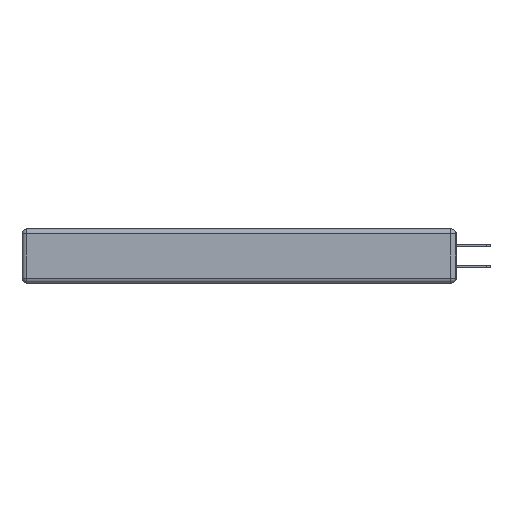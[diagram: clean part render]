
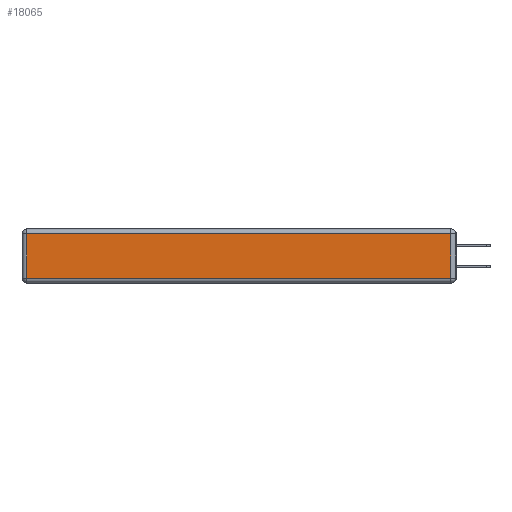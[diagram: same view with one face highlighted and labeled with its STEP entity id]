
A CAD part, left-side view. The second image highlights one B-rep face of the part: STEP entity #18065.
In plain terms, the highlighted planar face has unit normal (-1, 0, 0).
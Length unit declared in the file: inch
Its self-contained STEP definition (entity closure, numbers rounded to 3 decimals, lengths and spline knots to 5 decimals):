
#1673 = EDGE_LOOP ( 'NONE', ( #3307, #16689, #12419, #11632 ) ) ;
#2070 = DIRECTION ( 'NONE',  ( 0., 0., 1. ) ) ;
#2139 = EDGE_CURVE ( 'NONE', #7659, #4216, #4176, .T. ) ;
#2197 = FACE_OUTER_BOUND ( 'NONE', #1673, .T. ) ;
#2214 = LINE ( 'NONE', #5615, #16851 ) ;
#3307 = ORIENTED_EDGE ( 'NONE', *, *, #6347, .T. ) ;
#3391 = VERTEX_POINT ( 'NONE', #14250 ) ;
#4176 = LINE ( 'NONE', #8265, #8366 ) ;
#4216 = VERTEX_POINT ( 'NONE', #15046 ) ;
#5615 = CARTESIAN_POINT ( 'NONE',  ( 0., 2.75, -0.03 ) ) ;
#6186 = CARTESIAN_POINT ( 'NONE',  ( 0., 0., -0.343 ) ) ;
#6347 = EDGE_CURVE ( 'NONE', #4216, #3391, #11576, .T. ) ;
#6698 = VERTEX_POINT ( 'NONE', #11200 ) ;
#6755 = LINE ( 'NONE', #16153, #8767 ) ;
#7546 = PLANE ( 'NONE',  #13566 ) ;
#7659 = VERTEX_POINT ( 'NONE', #10006 ) ;
#8265 = CARTESIAN_POINT ( 'NONE',  ( 0., 2.72, -0.343 ) ) ;
#8366 = VECTOR ( 'NONE', #11650, 39.37008 ) ;
#8767 = VECTOR ( 'NONE', #2070, 39.37008 ) ;
#10004 = VECTOR ( 'NONE', #11533, 39.37008 ) ;
#10006 = CARTESIAN_POINT ( 'NONE',  ( 0., 2.72, -0.03 ) ) ;
#10333 = EDGE_CURVE ( 'NONE', #3391, #6698, #6755, .T. ) ;
#11200 = CARTESIAN_POINT ( 'NONE',  ( 0., 0.03, -0.03 ) ) ;
#11475 = CARTESIAN_POINT ( 'NONE',  ( 0., 0., -0.313 ) ) ;
#11533 = DIRECTION ( 'NONE',  ( 0., -1., 0. ) ) ;
#11576 = LINE ( 'NONE', #11475, #10004 ) ;
#11632 = ORIENTED_EDGE ( 'NONE', *, *, #2139, .T. ) ;
#11650 = DIRECTION ( 'NONE',  ( 0., 0., -1. ) ) ;
#12419 = ORIENTED_EDGE ( 'NONE', *, *, #17953, .T. ) ;
#13275 = DIRECTION ( 'NONE',  ( -1., 0., 0. ) ) ;
#13566 = AXIS2_PLACEMENT_3D ( 'NONE', #6186, #13275, #16279 ) ;
#14250 = CARTESIAN_POINT ( 'NONE',  ( 0., 0.03, -0.313 ) ) ;
#15046 = CARTESIAN_POINT ( 'NONE',  ( 0., 2.72, -0.313 ) ) ;
#16153 = CARTESIAN_POINT ( 'NONE',  ( 0., 0.03, -0.343 ) ) ;
#16279 = DIRECTION ( 'NONE',  ( 0., 0., 1. ) ) ;
#16689 = ORIENTED_EDGE ( 'NONE', *, *, #10333, .T. ) ;
#16851 = VECTOR ( 'NONE', #16941, 39.37008 ) ;
#16941 = DIRECTION ( 'NONE',  ( 0., 1., 0. ) ) ;
#17953 = EDGE_CURVE ( 'NONE', #6698, #7659, #2214, .T. ) ;
#18065 = ADVANCED_FACE ( 'NONE', ( #2197 ), #7546, .T. ) ;
